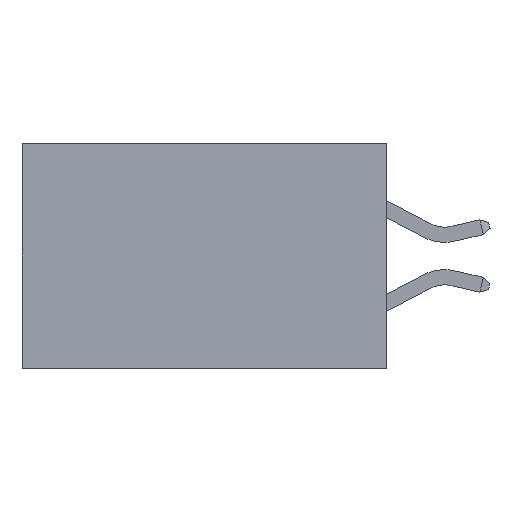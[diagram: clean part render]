
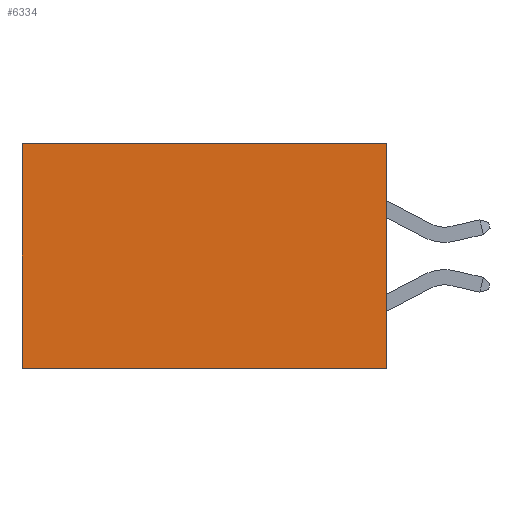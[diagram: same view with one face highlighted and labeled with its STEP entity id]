
A CAD part, left-side view. The second image highlights one B-rep face of the part: STEP entity #6334.
In plain terms, the highlighted planar face has unit normal (-1, 0, 0).
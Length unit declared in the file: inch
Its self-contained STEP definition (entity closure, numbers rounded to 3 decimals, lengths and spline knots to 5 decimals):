
#183 = EDGE_CURVE ( 'NONE', #7051, #1523, #14910, .T. ) ;
#539 = CARTESIAN_POINT ( 'NONE',  ( 0.298, 0.6, -0.37 ) ) ;
#739 = DIRECTION ( 'NONE',  ( 0., 0., -1. ) ) ;
#903 = DIRECTION ( 'NONE',  ( 1., 0., 0. ) ) ;
#964 = EDGE_LOOP ( 'NONE', ( #2283, #4684, #4398, #10059 ) ) ;
#1523 = VERTEX_POINT ( 'NONE', #539 ) ;
#1933 = PLANE ( 'NONE',  #16326 ) ;
#2161 = CARTESIAN_POINT ( 'NONE',  ( 0.298, 0.6, 0. ) ) ;
#2170 = CARTESIAN_POINT ( 'NONE',  ( 0.298, 0., 0. ) ) ;
#2277 = LINE ( 'NONE', #8409, #9050 ) ;
#2283 = ORIENTED_EDGE ( 'NONE', *, *, #183, .T. ) ;
#4398 = ORIENTED_EDGE ( 'NONE', *, *, #7840, .F. ) ;
#4601 = DIRECTION ( 'NONE',  ( 0., 1., 0. ) ) ;
#4684 = ORIENTED_EDGE ( 'NONE', *, *, #9732, .F. ) ;
#5182 = CARTESIAN_POINT ( 'NONE',  ( 0.298, 0., -0.37 ) ) ;
#5638 = CARTESIAN_POINT ( 'NONE',  ( 0.298, 0.6, 0. ) ) ;
#5940 = LINE ( 'NONE', #15864, #9612 ) ;
#6258 = FACE_OUTER_BOUND ( 'NONE', #964, .T. ) ;
#6334 = ADVANCED_FACE ( 'NONE', ( #6258 ), #1933, .F. ) ;
#7051 = VERTEX_POINT ( 'NONE', #2161 ) ;
#7840 = EDGE_CURVE ( 'NONE', #15198, #15725, #9885, .T. ) ;
#7861 = VECTOR ( 'NONE', #11103, 39.37008 ) ;
#8409 = CARTESIAN_POINT ( 'NONE',  ( 0.298, 0., 0. ) ) ;
#8770 = CARTESIAN_POINT ( 'NONE',  ( 0.298, 0., 0. ) ) ;
#9050 = VECTOR ( 'NONE', #15872, 39.37008 ) ;
#9529 = EDGE_CURVE ( 'NONE', #15198, #7051, #2277, .T. ) ;
#9612 = VECTOR ( 'NONE', #4601, 39.37008 ) ;
#9732 = EDGE_CURVE ( 'NONE', #15725, #1523, #5940, .T. ) ;
#9885 = LINE ( 'NONE', #8770, #12848 ) ;
#10059 = ORIENTED_EDGE ( 'NONE', *, *, #9529, .T. ) ;
#10669 = CARTESIAN_POINT ( 'NONE',  ( 0.298, 0., 0. ) ) ;
#11103 = DIRECTION ( 'NONE',  ( 0., 0., -1. ) ) ;
#12536 = DIRECTION ( 'NONE',  ( 0., 0., -1. ) ) ;
#12848 = VECTOR ( 'NONE', #12536, 39.37008 ) ;
#14910 = LINE ( 'NONE', #5638, #7861 ) ;
#15198 = VERTEX_POINT ( 'NONE', #10669 ) ;
#15725 = VERTEX_POINT ( 'NONE', #5182 ) ;
#15864 = CARTESIAN_POINT ( 'NONE',  ( 0.298, 0., -0.37 ) ) ;
#15872 = DIRECTION ( 'NONE',  ( 0., 1., 0. ) ) ;
#16326 = AXIS2_PLACEMENT_3D ( 'NONE', #2170, #903, #739 ) ;
